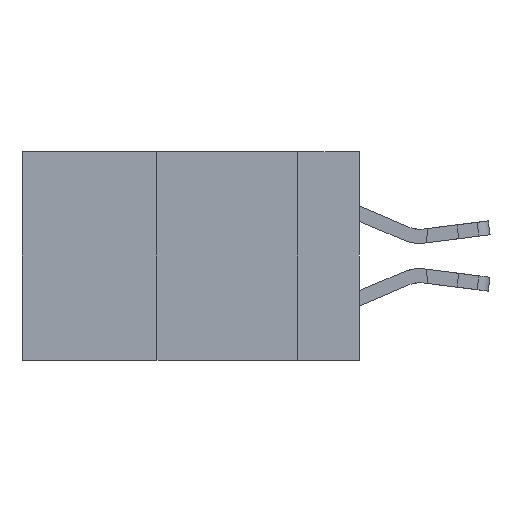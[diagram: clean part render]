
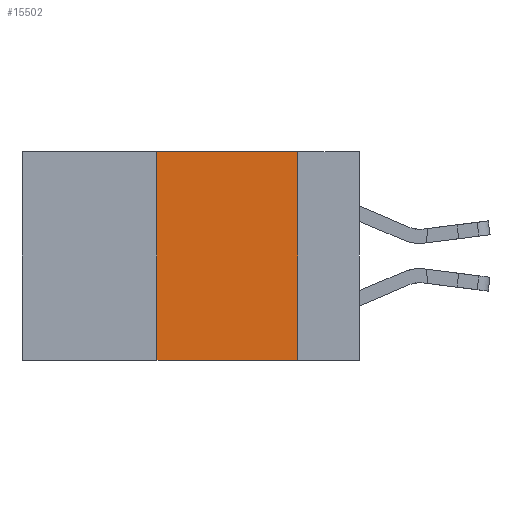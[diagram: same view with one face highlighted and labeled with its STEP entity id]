
A CAD part, left-side view. The second image highlights one B-rep face of the part: STEP entity #15502.
In plain terms, the highlighted planar face has unit normal (-1, 0, 0).
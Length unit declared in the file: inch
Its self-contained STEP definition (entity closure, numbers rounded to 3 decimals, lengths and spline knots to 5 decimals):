
#629 = EDGE_CURVE ( 'NONE', #8402, #14320, #11945, .T. ) ;
#2354 = LINE ( 'NONE', #7140, #19605 ) ;
#2642 = FACE_OUTER_BOUND ( 'NONE', #12668, .T. ) ;
#3303 = ORIENTED_EDGE ( 'NONE', *, *, #13535, .F. ) ;
#4208 = DIRECTION ( 'NONE',  ( 0., 0., -1. ) ) ;
#4250 = CARTESIAN_POINT ( 'NONE',  ( 0., 0.6, -0.37 ) ) ;
#4352 = DIRECTION ( 'NONE',  ( 0., -1., 0. ) ) ;
#4374 = VECTOR ( 'NONE', #10675, 39.37008 ) ;
#4429 = CARTESIAN_POINT ( 'NONE',  ( 0., 0.6, 0. ) ) ;
#4553 = CARTESIAN_POINT ( 'NONE',  ( 0., 0.11, -0.37 ) ) ;
#4732 = LINE ( 'NONE', #4429, #4374 ) ;
#6705 = ORIENTED_EDGE ( 'NONE', *, *, #20161, .F. ) ;
#6949 = ORIENTED_EDGE ( 'NONE', *, *, #629, .T. ) ;
#7140 = CARTESIAN_POINT ( 'NONE',  ( 0., 0.36, 0. ) ) ;
#7234 = CARTESIAN_POINT ( 'NONE',  ( 0., 0.6, 0. ) ) ;
#8402 = VERTEX_POINT ( 'NONE', #18082 ) ;
#8881 = DIRECTION ( 'NONE',  ( 1., 0., 0. ) ) ;
#9582 = VECTOR ( 'NONE', #4352, 39.37008 ) ;
#10675 = DIRECTION ( 'NONE',  ( 0., -1., 0. ) ) ;
#11184 = AXIS2_PLACEMENT_3D ( 'NONE', #7234, #8881, #18065 ) ;
#11386 = CARTESIAN_POINT ( 'NONE',  ( 0., 0.36, 0. ) ) ;
#11761 = PLANE ( 'NONE',  #11184 ) ;
#11945 = LINE ( 'NONE', #4250, #9582 ) ;
#12668 = EDGE_LOOP ( 'NONE', ( #6705, #3303, #15732, #6949 ) ) ;
#13535 = EDGE_CURVE ( 'NONE', #16805, #15557, #4732, .T. ) ;
#13697 = DIRECTION ( 'NONE',  ( 0., 0., 1. ) ) ;
#14189 = VECTOR ( 'NONE', #4208, 39.37008 ) ;
#14320 = VERTEX_POINT ( 'NONE', #4553 ) ;
#14923 = CARTESIAN_POINT ( 'NONE',  ( 0., 0.11, 0. ) ) ;
#14949 = CARTESIAN_POINT ( 'NONE',  ( 0., 0.11, 0. ) ) ;
#15502 = ADVANCED_FACE ( 'NONE', ( #2642 ), #11761, .F. ) ;
#15557 = VERTEX_POINT ( 'NONE', #14923 ) ;
#15732 = ORIENTED_EDGE ( 'NONE', *, *, #16922, .F. ) ;
#16805 = VERTEX_POINT ( 'NONE', #11386 ) ;
#16922 = EDGE_CURVE ( 'NONE', #8402, #16805, #2354, .T. ) ;
#18065 = DIRECTION ( 'NONE',  ( 0., 0., -1. ) ) ;
#18082 = CARTESIAN_POINT ( 'NONE',  ( 0., 0.36, -0.37 ) ) ;
#19605 = VECTOR ( 'NONE', #13697, 39.37008 ) ;
#19926 = LINE ( 'NONE', #14949, #14189 ) ;
#20161 = EDGE_CURVE ( 'NONE', #15557, #14320, #19926, .T. ) ;
